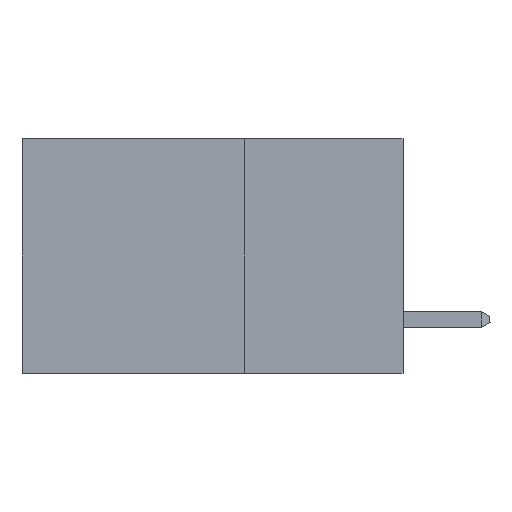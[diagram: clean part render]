
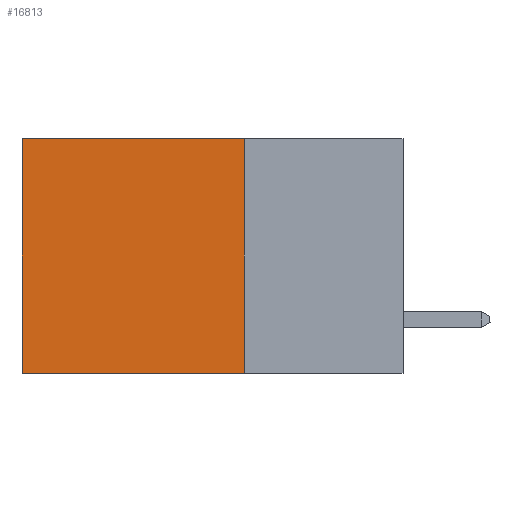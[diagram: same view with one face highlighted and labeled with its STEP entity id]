
A CAD part, left-side view. The second image highlights one B-rep face of the part: STEP entity #16813.
In plain terms, the highlighted planar face has unit normal (-1, 0, 0).
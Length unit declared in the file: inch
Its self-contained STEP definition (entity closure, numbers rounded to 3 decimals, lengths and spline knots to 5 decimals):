
#358 = DIRECTION ( 'NONE',  ( 1., 0., 0. ) ) ;
#428 = VECTOR ( 'NONE', #4643, 39.37008 ) ;
#2030 = VERTEX_POINT ( 'NONE', #25392 ) ;
#2476 = ORIENTED_EDGE ( 'NONE', *, *, #11355, .T. ) ;
#4643 = DIRECTION ( 'NONE',  ( 0., 1., 0. ) ) ;
#5023 = VERTEX_POINT ( 'NONE', #20072 ) ;
#5115 = VECTOR ( 'NONE', #24238, 39.37008 ) ;
#7038 = VECTOR ( 'NONE', #11731, 39.37008 ) ;
#7829 = FACE_OUTER_BOUND ( 'NONE', #12426, .T. ) ;
#8938 = ORIENTED_EDGE ( 'NONE', *, *, #13365, .T. ) ;
#9111 = AXIS2_PLACEMENT_3D ( 'NONE', #16713, #358, #22955 ) ;
#9648 = CARTESIAN_POINT ( 'NONE',  ( 0.2875, 0.25, 0. ) ) ;
#11292 = DIRECTION ( 'NONE',  ( 0., 1., 0. ) ) ;
#11355 = EDGE_CURVE ( 'NONE', #2030, #5023, #25757, .T. ) ;
#11731 = DIRECTION ( 'NONE',  ( 0., 0., -1. ) ) ;
#12188 = VECTOR ( 'NONE', #11292, 39.37008 ) ;
#12309 = VERTEX_POINT ( 'NONE', #24737 ) ;
#12426 = EDGE_LOOP ( 'NONE', ( #2476, #19688, #19222, #8938 ) ) ;
#12677 = PLANE ( 'NONE',  #9111 ) ;
#12846 = CARTESIAN_POINT ( 'NONE',  ( 0.2875, 0.25, -0.37 ) ) ;
#13365 = EDGE_CURVE ( 'NONE', #12309, #2030, #17675, .T. ) ;
#15519 = CARTESIAN_POINT ( 'NONE',  ( 0.2875, 0.25, 0. ) ) ;
#16713 = CARTESIAN_POINT ( 'NONE',  ( 0.2875, 0.25, 0. ) ) ;
#16813 = ADVANCED_FACE ( 'NONE', ( #7829 ), #12677, .F. ) ;
#16971 = EDGE_CURVE ( 'NONE', #24640, #5023, #25226, .T. ) ;
#17675 = LINE ( 'NONE', #15519, #12188 ) ;
#18240 = CARTESIAN_POINT ( 'NONE',  ( 0.2875, 0.25, -0.37 ) ) ;
#19222 = ORIENTED_EDGE ( 'NONE', *, *, #20024, .F. ) ;
#19688 = ORIENTED_EDGE ( 'NONE', *, *, #16971, .F. ) ;
#20024 = EDGE_CURVE ( 'NONE', #12309, #24640, #24790, .T. ) ;
#20072 = CARTESIAN_POINT ( 'NONE',  ( 0.2875, 0.6, -0.37 ) ) ;
#20097 = CARTESIAN_POINT ( 'NONE',  ( 0.2875, 0.6, 0. ) ) ;
#22955 = DIRECTION ( 'NONE',  ( 0., 0., -1. ) ) ;
#24238 = DIRECTION ( 'NONE',  ( 0., 0., -1. ) ) ;
#24640 = VERTEX_POINT ( 'NONE', #18240 ) ;
#24737 = CARTESIAN_POINT ( 'NONE',  ( 0.2875, 0.25, 0. ) ) ;
#24790 = LINE ( 'NONE', #9648, #7038 ) ;
#25226 = LINE ( 'NONE', #12846, #428 ) ;
#25392 = CARTESIAN_POINT ( 'NONE',  ( 0.2875, 0.6, 0. ) ) ;
#25757 = LINE ( 'NONE', #20097, #5115 ) ;
